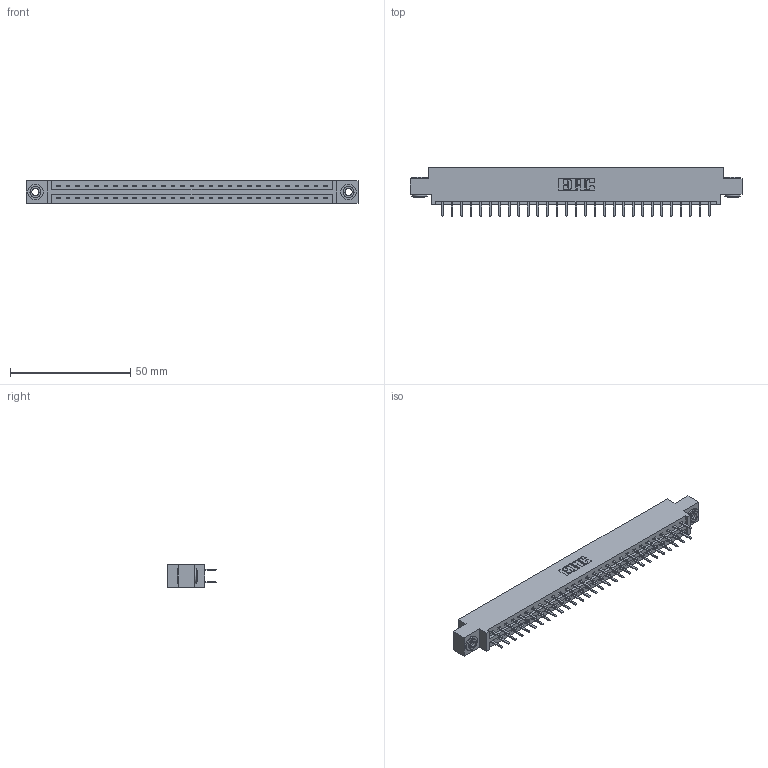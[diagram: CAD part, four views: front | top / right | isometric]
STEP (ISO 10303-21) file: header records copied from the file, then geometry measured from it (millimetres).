
FILE_DESCRIPTION (( 'STEP AP203' ), '1' );
FILE_NAME ('387-058-520-803.STEP', '2019-10-19T08:22:08', ( '' ), ( '' ), 'SwSTEP 2.0', 'SolidWorks 2016', '' );
FILE_SCHEMA (( 'CONFIG_CONTROL_DESIGN' ));
Length unit declared in the file: inch
Products named in the file (4): 337 Part_0.170 Offset - 0.156 Dia-TH; 345-292-001_345-293-120; 345-250-002_345-250-002-102; 387-058-520-803
Assembly tree (61 placements, depth 2):
  387-058-520-803
    337 Part_0.170 Offset - 0.156 Dia-TH
    345-292-001_345-293-120  x58
    345-250-002_345-250-002-102  x2
Bounding box: 137.92 x 20.02 x 9.4 mm (x, y, z)
Volume: 14238.7 mm3; surface area: 16230.1 mm2
Topology: 61 solids, 61 shells, 3520 faces, 10201 edges, 6642 vertices
Faces by surface type: plane 2404, cylinder 1108, cone 8
Entity records: 25062 total; most frequent: CARTESIAN_POINT 4221, ORIENTED_EDGE 4138, DIRECTION 3635, EDGE_CURVE 2069, LINE 1913, VECTOR 1913, VERTEX_POINT 1374, AXIS2_PLACEMENT_3D 861
